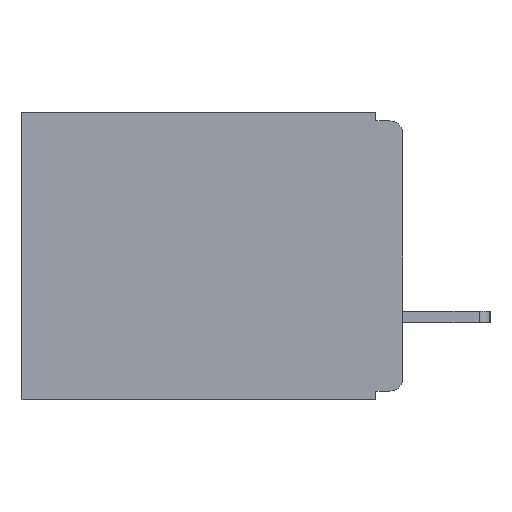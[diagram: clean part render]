
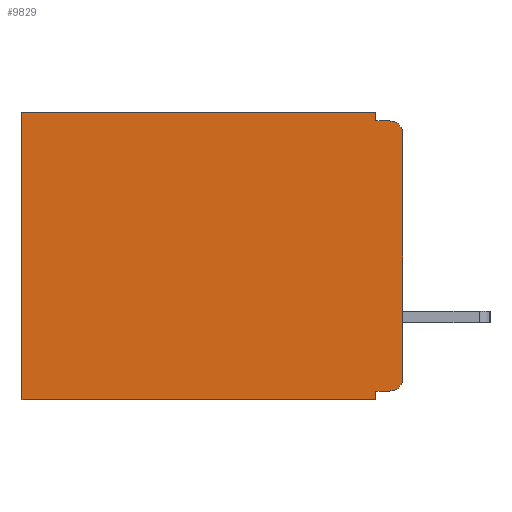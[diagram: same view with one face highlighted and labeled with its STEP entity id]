
A CAD part, left-side view. The second image highlights one B-rep face of the part: STEP entity #9829.
In plain terms, the highlighted planar face has unit normal (-1, 0, 0).
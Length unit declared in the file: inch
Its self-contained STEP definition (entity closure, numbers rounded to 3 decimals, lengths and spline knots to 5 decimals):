
#447 = CARTESIAN_POINT ( 'NONE',  ( 0.3, 0.015, -0.32 ) ) ;
#655 = EDGE_CURVE ( 'NONE', #6993, #18775, #28000, .T. ) ;
#664 = CARTESIAN_POINT ( 'NONE',  ( 0.3, 0., -0.01 ) ) ;
#1144 = EDGE_CURVE ( 'NONE', #12889, #23491, #27675, .T. ) ;
#1587 = ORIENTED_EDGE ( 'NONE', *, *, #27267, .F. ) ;
#1854 = FACE_OUTER_BOUND ( 'NONE', #5218, .T. ) ;
#1994 = CARTESIAN_POINT ( 'NONE',  ( 0.3, 0.031, 0. ) ) ;
#2042 = ORIENTED_EDGE ( 'NONE', *, *, #1144, .T. ) ;
#2056 = DIRECTION ( 'NONE',  ( -1., 0., 0. ) ) ;
#2320 = CARTESIAN_POINT ( 'NONE',  ( 0.3, 0.031, -0.32 ) ) ;
#2371 = ORIENTED_EDGE ( 'NONE', *, *, #655, .T. ) ;
#3072 = VERTEX_POINT ( 'NONE', #24600 ) ;
#3952 = CARTESIAN_POINT ( 'NONE',  ( 0.3, 0., -0.32 ) ) ;
#4115 = DIRECTION ( 'NONE',  ( 0., 1., 0. ) ) ;
#4685 = VECTOR ( 'NONE', #23402, 39.37008 ) ;
#4813 = LINE ( 'NONE', #15702, #29669 ) ;
#4832 = CARTESIAN_POINT ( 'NONE',  ( 0.3, 0.031, -0.33 ) ) ;
#5156 = AXIS2_PLACEMENT_3D ( 'NONE', #9132, #21733, #7187 ) ;
#5218 = EDGE_LOOP ( 'NONE', ( #27190, #2042, #7685, #11143, #27135, #2371, #1587, #28364, #19548, #8938 ) ) ;
#5442 = LINE ( 'NONE', #11784, #4685 ) ;
#6187 = DIRECTION ( 'NONE',  ( 0., 0., -1. ) ) ;
#6359 = CARTESIAN_POINT ( 'NONE',  ( 0.3, 0.031, -0.33 ) ) ;
#6993 = VERTEX_POINT ( 'NONE', #29047 ) ;
#7187 = DIRECTION ( 'NONE',  ( 0., 0., -1. ) ) ;
#7685 = ORIENTED_EDGE ( 'NONE', *, *, #23247, .F. ) ;
#7804 = DIRECTION ( 'NONE',  ( 0., -1., 0. ) ) ;
#8395 = CARTESIAN_POINT ( 'NONE',  ( 0.3, 0.031, -0.01 ) ) ;
#8517 = EDGE_CURVE ( 'NONE', #23738, #8596, #20044, .T. ) ;
#8596 = VERTEX_POINT ( 'NONE', #4832 ) ;
#8938 = ORIENTED_EDGE ( 'NONE', *, *, #25383, .T. ) ;
#9132 = CARTESIAN_POINT ( 'NONE',  ( 0.3, 0.015, -0.025 ) ) ;
#9829 = ADVANCED_FACE ( 'NONE', ( #1854 ), #23913, .F. ) ;
#10185 = EDGE_CURVE ( 'NONE', #21074, #6993, #4813, .T. ) ;
#10735 = EDGE_CURVE ( 'NONE', #18813, #23738, #15541, .T. ) ;
#11048 = CARTESIAN_POINT ( 'NONE',  ( 0.3, 0.031, 0. ) ) ;
#11143 = ORIENTED_EDGE ( 'NONE', *, *, #11666, .F. ) ;
#11666 = EDGE_CURVE ( 'NONE', #21074, #13381, #13274, .T. ) ;
#11726 = EDGE_CURVE ( 'NONE', #12889, #3072, #5442, .T. ) ;
#11784 = CARTESIAN_POINT ( 'NONE',  ( 0.3, 0., -0.33 ) ) ;
#12527 = VECTOR ( 'NONE', #27831, 39.37008 ) ;
#12889 = VERTEX_POINT ( 'NONE', #29857 ) ;
#13274 = LINE ( 'NONE', #1994, #12527 ) ;
#13381 = VERTEX_POINT ( 'NONE', #8395 ) ;
#14725 = CARTESIAN_POINT ( 'NONE',  ( 0.3, 0.437, -0.33 ) ) ;
#14967 = AXIS2_PLACEMENT_3D ( 'NONE', #16261, #2056, #18594 ) ;
#15541 = LINE ( 'NONE', #3952, #27828 ) ;
#15702 = CARTESIAN_POINT ( 'NONE',  ( 0.3, 0., 0. ) ) ;
#15707 = DIRECTION ( 'NONE',  ( 0., 1., 0. ) ) ;
#15713 = VECTOR ( 'NONE', #17671, 39.37008 ) ;
#16261 = CARTESIAN_POINT ( 'NONE',  ( 0.3, 0.015, -0.305 ) ) ;
#16748 = LINE ( 'NONE', #16768, #28331 ) ;
#16768 = CARTESIAN_POINT ( 'NONE',  ( 0.3, 0., -0.33 ) ) ;
#17671 = DIRECTION ( 'NONE',  ( 0., 0., -1. ) ) ;
#18594 = DIRECTION ( 'NONE',  ( 0., 0., -1. ) ) ;
#18775 = VERTEX_POINT ( 'NONE', #14725 ) ;
#18813 = VERTEX_POINT ( 'NONE', #447 ) ;
#19099 = DIRECTION ( 'NONE',  ( 0., 1., 0. ) ) ;
#19548 = ORIENTED_EDGE ( 'NONE', *, *, #10735, .F. ) ;
#20044 = LINE ( 'NONE', #6359, #25478 ) ;
#20296 = CARTESIAN_POINT ( 'NONE',  ( 0.3, 0.015, -0.01 ) ) ;
#21074 = VERTEX_POINT ( 'NONE', #11048 ) ;
#21733 = DIRECTION ( 'NONE',  ( -1., 0., 0. ) ) ;
#22425 = VECTOR ( 'NONE', #7804, 39.37008 ) ;
#23139 = LINE ( 'NONE', #664, #22425 ) ;
#23247 = EDGE_CURVE ( 'NONE', #13381, #23491, #23139, .T. ) ;
#23402 = DIRECTION ( 'NONE',  ( 0., 0., -1. ) ) ;
#23491 = VERTEX_POINT ( 'NONE', #20296 ) ;
#23558 = DIRECTION ( 'NONE',  ( 0., 0., -1. ) ) ;
#23655 = DIRECTION ( 'NONE',  ( 1., 0., 0. ) ) ;
#23689 = CARTESIAN_POINT ( 'NONE',  ( 0.3, 0., -0.33 ) ) ;
#23738 = VERTEX_POINT ( 'NONE', #2320 ) ;
#23913 = PLANE ( 'NONE',  #27818 ) ;
#24600 = CARTESIAN_POINT ( 'NONE',  ( 0.3, 0., -0.305 ) ) ;
#25383 = EDGE_CURVE ( 'NONE', #18813, #3072, #27684, .T. ) ;
#25455 = CARTESIAN_POINT ( 'NONE',  ( 0.3, 0.437, -0.33 ) ) ;
#25478 = VECTOR ( 'NONE', #6187, 39.37008 ) ;
#27135 = ORIENTED_EDGE ( 'NONE', *, *, #10185, .T. ) ;
#27190 = ORIENTED_EDGE ( 'NONE', *, *, #11726, .F. ) ;
#27267 = EDGE_CURVE ( 'NONE', #8596, #18775, #16748, .T. ) ;
#27675 = CIRCLE ( 'NONE', #5156, 0.015 ) ;
#27684 = CIRCLE ( 'NONE', #14967, 0.015 ) ;
#27818 = AXIS2_PLACEMENT_3D ( 'NONE', #23689, #23655, #23558 ) ;
#27828 = VECTOR ( 'NONE', #4115, 39.37008 ) ;
#27831 = DIRECTION ( 'NONE',  ( 0., 0., -1. ) ) ;
#28000 = LINE ( 'NONE', #25455, #15713 ) ;
#28331 = VECTOR ( 'NONE', #19099, 39.37008 ) ;
#28364 = ORIENTED_EDGE ( 'NONE', *, *, #8517, .F. ) ;
#29047 = CARTESIAN_POINT ( 'NONE',  ( 0.3, 0.437, 0. ) ) ;
#29669 = VECTOR ( 'NONE', #15707, 39.37008 ) ;
#29857 = CARTESIAN_POINT ( 'NONE',  ( 0.3, 0., -0.025 ) ) ;
